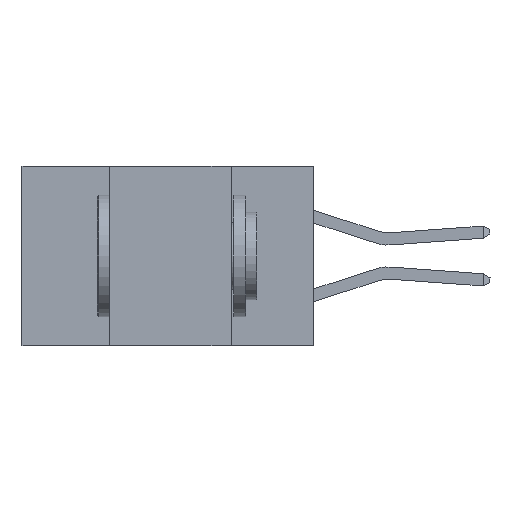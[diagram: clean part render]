
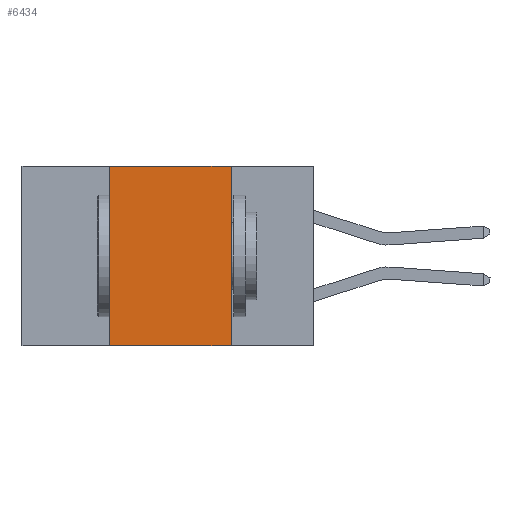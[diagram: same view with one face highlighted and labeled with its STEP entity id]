
A CAD part, left-side view. The second image highlights one B-rep face of the part: STEP entity #6434.
In plain terms, the highlighted planar face has unit normal (-1, 0, 0).
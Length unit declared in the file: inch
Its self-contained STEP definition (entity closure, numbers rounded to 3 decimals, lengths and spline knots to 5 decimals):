
#539 = CARTESIAN_POINT ( 'NONE',  ( 0., 0.42, 0. ) ) ;
#707 = DIRECTION ( 'NONE',  ( 0., 0., -1. ) ) ;
#727 = LINE ( 'NONE', #9143, #2391 ) ;
#961 = VECTOR ( 'NONE', #6236, 39.37008 ) ;
#1491 = AXIS2_PLACEMENT_3D ( 'NONE', #4590, #5447, #2256 ) ;
#2049 = VERTEX_POINT ( 'NONE', #5312 ) ;
#2256 = DIRECTION ( 'NONE',  ( 0., 0., -1. ) ) ;
#2391 = VECTOR ( 'NONE', #4371, 39.37008 ) ;
#2553 = EDGE_CURVE ( 'NONE', #2049, #8551, #5902, .T. ) ;
#2737 = CARTESIAN_POINT ( 'NONE',  ( 0., 0.6, 0. ) ) ;
#3471 = EDGE_CURVE ( 'NONE', #8551, #7255, #6490, .T. ) ;
#3514 = DIRECTION ( 'NONE',  ( 0., -1., 0. ) ) ;
#4345 = VECTOR ( 'NONE', #3514, 39.37008 ) ;
#4371 = DIRECTION ( 'NONE',  ( 0., -1., 0. ) ) ;
#4590 = CARTESIAN_POINT ( 'NONE',  ( 0., 0.6, 0. ) ) ;
#4766 = CARTESIAN_POINT ( 'NONE',  ( 0., 0.17, 0. ) ) ;
#5276 = CARTESIAN_POINT ( 'NONE',  ( 0., 0.42, -0.37 ) ) ;
#5312 = CARTESIAN_POINT ( 'NONE',  ( 0., 0.42, 0. ) ) ;
#5371 = EDGE_CURVE ( 'NONE', #9345, #7255, #727, .T. ) ;
#5447 = DIRECTION ( 'NONE',  ( 1., 0., 0. ) ) ;
#5584 = CARTESIAN_POINT ( 'NONE',  ( 0., 0.17, 0. ) ) ;
#5873 = VECTOR ( 'NONE', #707, 39.37008 ) ;
#5902 = LINE ( 'NONE', #2737, #4345 ) ;
#6236 = DIRECTION ( 'NONE',  ( 0., 0., 1. ) ) ;
#6275 = EDGE_CURVE ( 'NONE', #9345, #2049, #8920, .T. ) ;
#6434 = ADVANCED_FACE ( 'NONE', ( #7169 ), #7045, .F. ) ;
#6490 = LINE ( 'NONE', #5584, #5873 ) ;
#7045 = PLANE ( 'NONE',  #1491 ) ;
#7169 = FACE_OUTER_BOUND ( 'NONE', #7450, .T. ) ;
#7215 = CARTESIAN_POINT ( 'NONE',  ( 0., 0.17, -0.37 ) ) ;
#7255 = VERTEX_POINT ( 'NONE', #7215 ) ;
#7450 = EDGE_LOOP ( 'NONE', ( #9325, #9803, #10001, #9749 ) ) ;
#8551 = VERTEX_POINT ( 'NONE', #4766 ) ;
#8920 = LINE ( 'NONE', #539, #961 ) ;
#9143 = CARTESIAN_POINT ( 'NONE',  ( 0., 0.6, -0.37 ) ) ;
#9325 = ORIENTED_EDGE ( 'NONE', *, *, #3471, .F. ) ;
#9345 = VERTEX_POINT ( 'NONE', #5276 ) ;
#9749 = ORIENTED_EDGE ( 'NONE', *, *, #5371, .T. ) ;
#9803 = ORIENTED_EDGE ( 'NONE', *, *, #2553, .F. ) ;
#10001 = ORIENTED_EDGE ( 'NONE', *, *, #6275, .F. ) ;
